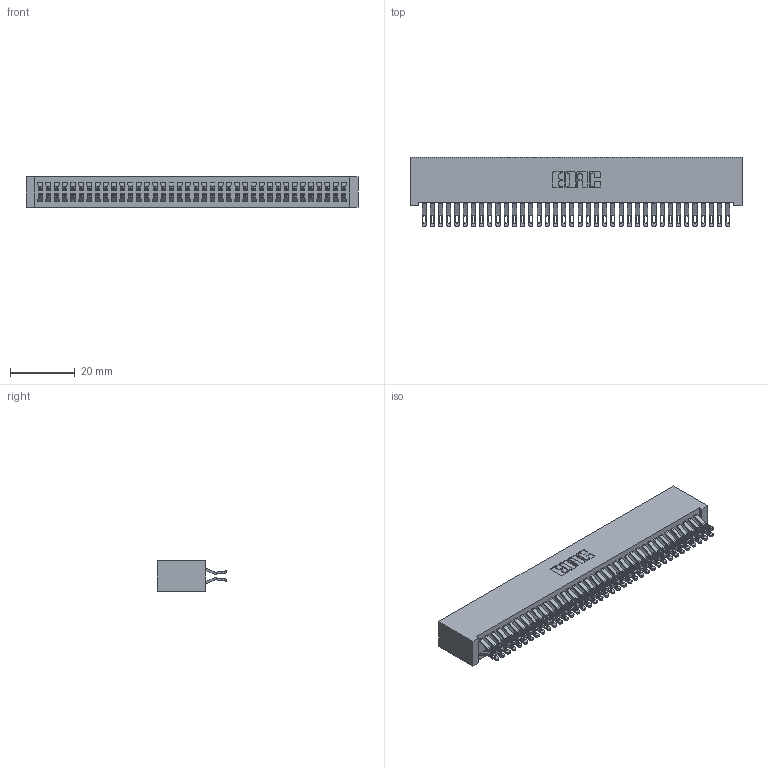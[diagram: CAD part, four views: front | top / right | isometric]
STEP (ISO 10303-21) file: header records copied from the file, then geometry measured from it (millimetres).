
FILE_DESCRIPTION (( 'STEP AP203' ), '1' );
FILE_NAME ('342-076-555-201.STEP', '2018-08-13T12:38:02', ( '' ), ( '' ), 'SwSTEP 2.0', 'SolidWorks 2016', '' );
FILE_SCHEMA (( 'CONFIG_CONTROL_DESIGN' ));
Length unit declared in the file: inch
Products named in the file (3): 342-076-555-201; 342 Part_Lugless; 345-292-001_555 Tail
Assembly tree (77 placements, depth 2):
  342-076-555-201
    342 Part_Lugless
    345-292-001_555 Tail  x76
Bounding box: 102.77 x 21.47 x 9.4 mm (x, y, z)
Volume: 9865.5 mm3; surface area: 17141.6 mm2
Topology: 77 solids, 77 shells, 4510 faces, 14183 edges, 9454 vertices
Faces by surface type: plane 2646, cylinder 1864
Entity records: 24881 total; most frequent: CARTESIAN_POINT 4160, ORIENTED_EDGE 4066, DIRECTION 3525, EDGE_CURVE 2033, LINE 1893, VECTOR 1893, VERTEX_POINT 1354, AXIS2_PLACEMENT_3D 816
